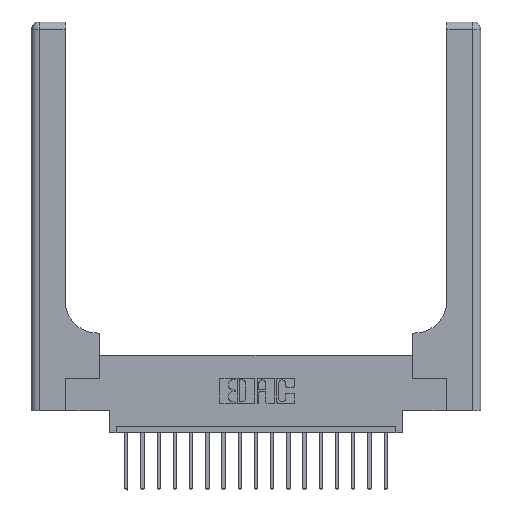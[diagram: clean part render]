
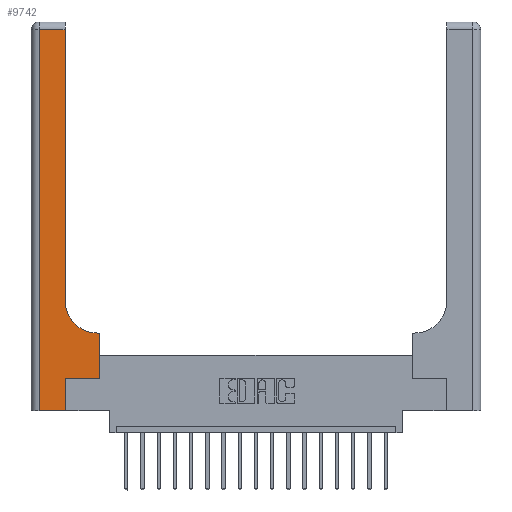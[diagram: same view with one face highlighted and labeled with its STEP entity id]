
A CAD part, top view. The second image highlights one B-rep face of the part: STEP entity #9742.
In plain terms, the highlighted planar face has unit normal (0, 0, 1).
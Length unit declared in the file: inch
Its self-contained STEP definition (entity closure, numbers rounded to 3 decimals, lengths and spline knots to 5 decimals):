
#14 = ORIENTED_EDGE ( 'NONE', *, *, #11265, .T. ) ;
#699 = DIRECTION ( 'NONE',  ( 0., 1., 0. ) ) ;
#896 = EDGE_LOOP ( 'NONE', ( #10444, #14141, #12593, #3415, #11266, #14292, #16196, #1144, #14 ) ) ;
#1080 = CARTESIAN_POINT ( 'NONE',  ( 0.265, 0.25, 0.37 ) ) ;
#1144 = ORIENTED_EDGE ( 'NONE', *, *, #6530, .T. ) ;
#1337 = VERTEX_POINT ( 'NONE', #7347 ) ;
#1409 = DIRECTION ( 'NONE',  ( 0., 1., 0. ) ) ;
#1794 = LINE ( 'NONE', #13833, #18723 ) ;
#1955 = CARTESIAN_POINT ( 'NONE',  ( 0.265, 0.25, 0.37 ) ) ;
#2036 = DIRECTION ( 'NONE',  ( -1., 0., 0. ) ) ;
#2071 = CARTESIAN_POINT ( 'NONE',  ( 0.26, 0.85, 0.37 ) ) ;
#2111 = LINE ( 'NONE', #3365, #17397 ) ;
#2700 = DIRECTION ( 'NONE',  ( 1., 0., 0. ) ) ;
#2970 = DIRECTION ( 'NONE',  ( 0., 1., 0. ) ) ;
#3365 = CARTESIAN_POINT ( 'NONE',  ( 0.528, 0.25, 0.37 ) ) ;
#3415 = ORIENTED_EDGE ( 'NONE', *, *, #11707, .T. ) ;
#3661 = LINE ( 'NONE', #10349, #5265 ) ;
#3766 = VECTOR ( 'NONE', #2700, 39.37008 ) ;
#4143 = EDGE_CURVE ( 'NONE', #1337, #18345, #2111, .T. ) ;
#4400 = CARTESIAN_POINT ( 'NONE',  ( 0.26, 2.94, 0.37 ) ) ;
#4460 = CIRCLE ( 'NONE', #9189, 0.25 ) ;
#4573 = LINE ( 'NONE', #12060, #5502 ) ;
#4612 = DIRECTION ( 'NONE',  ( 1., 0., 0. ) ) ;
#5010 = EDGE_CURVE ( 'NONE', #18431, #18228, #11331, .T. ) ;
#5265 = VECTOR ( 'NONE', #2970, 39.37008 ) ;
#5502 = VECTOR ( 'NONE', #13652, 39.37008 ) ;
#5650 = VERTEX_POINT ( 'NONE', #1080 ) ;
#5975 = EDGE_CURVE ( 'NONE', #5650, #1337, #9166, .T. ) ;
#6398 = CARTESIAN_POINT ( 'NONE',  ( 0.528, 0.6, 0.37 ) ) ;
#6530 = EDGE_CURVE ( 'NONE', #18345, #8696, #1794, .T. ) ;
#7207 = VERTEX_POINT ( 'NONE', #2071 ) ;
#7347 = CARTESIAN_POINT ( 'NONE',  ( 0.528, 0.25, 0.37 ) ) ;
#7786 = DIRECTION ( 'NONE',  ( -1., 0., 0. ) ) ;
#7935 = DIRECTION ( 'NONE',  ( 0., 0., -1. ) ) ;
#8696 = VERTEX_POINT ( 'NONE', #18028 ) ;
#8788 = EDGE_CURVE ( 'NONE', #7207, #14995, #3661, .T. ) ;
#9166 = LINE ( 'NONE', #1955, #10111 ) ;
#9174 = PLANE ( 'NONE',  #14900 ) ;
#9189 = AXIS2_PLACEMENT_3D ( 'NONE', #11883, #16386, #4612 ) ;
#9742 = ADVANCED_FACE ( 'NONE', ( #14523 ), #9174, .F. ) ;
#10111 = VECTOR ( 'NONE', #12582, 39.37008 ) ;
#10155 = CARTESIAN_POINT ( 'NONE',  ( 0.06, 2.94, 0.37 ) ) ;
#10349 = CARTESIAN_POINT ( 'NONE',  ( 0.26, 3., 0.37 ) ) ;
#10444 = ORIENTED_EDGE ( 'NONE', *, *, #8788, .T. ) ;
#10615 = VECTOR ( 'NONE', #13800, 39.37008 ) ;
#11148 = CARTESIAN_POINT ( 'NONE',  ( 0., 3., 0.37 ) ) ;
#11265 = EDGE_CURVE ( 'NONE', #8696, #7207, #4460, .T. ) ;
#11266 = ORIENTED_EDGE ( 'NONE', *, *, #18206, .T. ) ;
#11331 = LINE ( 'NONE', #12019, #10615 ) ;
#11529 = VERTEX_POINT ( 'NONE', #13926 ) ;
#11707 = EDGE_CURVE ( 'NONE', #18228, #11529, #14044, .T. ) ;
#11883 = CARTESIAN_POINT ( 'NONE',  ( 0.51, 0.85, 0.37 ) ) ;
#12019 = CARTESIAN_POINT ( 'NONE',  ( 0.06, 3., 0.37 ) ) ;
#12060 = CARTESIAN_POINT ( 'NONE',  ( 0., 2.94, 0.37 ) ) ;
#12582 = DIRECTION ( 'NONE',  ( 1., 0., 0. ) ) ;
#12593 = ORIENTED_EDGE ( 'NONE', *, *, #5010, .T. ) ;
#12853 = VECTOR ( 'NONE', #1409, 39.37008 ) ;
#13046 = CARTESIAN_POINT ( 'NONE',  ( 0., 0., 0.37 ) ) ;
#13652 = DIRECTION ( 'NONE',  ( -1., 0., 0. ) ) ;
#13800 = DIRECTION ( 'NONE',  ( 0., -1., 0. ) ) ;
#13833 = CARTESIAN_POINT ( 'NONE',  ( 0.26, 0.6, 0.37 ) ) ;
#13926 = CARTESIAN_POINT ( 'NONE',  ( 0.265, 0., 0.37 ) ) ;
#14044 = LINE ( 'NONE', #13046, #3766 ) ;
#14141 = ORIENTED_EDGE ( 'NONE', *, *, #14403, .T. ) ;
#14292 = ORIENTED_EDGE ( 'NONE', *, *, #5975, .T. ) ;
#14403 = EDGE_CURVE ( 'NONE', #14995, #18431, #4573, .T. ) ;
#14523 = FACE_OUTER_BOUND ( 'NONE', #896, .T. ) ;
#14701 = CARTESIAN_POINT ( 'NONE',  ( 0.265, 0., 0.37 ) ) ;
#14900 = AXIS2_PLACEMENT_3D ( 'NONE', #11148, #7935, #2036 ) ;
#14995 = VERTEX_POINT ( 'NONE', #4400 ) ;
#15112 = CARTESIAN_POINT ( 'NONE',  ( 0.06, 0., 0.37 ) ) ;
#15382 = LINE ( 'NONE', #14701, #12853 ) ;
#16196 = ORIENTED_EDGE ( 'NONE', *, *, #4143, .T. ) ;
#16386 = DIRECTION ( 'NONE',  ( 0., 0., -1. ) ) ;
#17397 = VECTOR ( 'NONE', #699, 39.37008 ) ;
#18028 = CARTESIAN_POINT ( 'NONE',  ( 0.51, 0.6, 0.37 ) ) ;
#18206 = EDGE_CURVE ( 'NONE', #11529, #5650, #15382, .T. ) ;
#18228 = VERTEX_POINT ( 'NONE', #15112 ) ;
#18345 = VERTEX_POINT ( 'NONE', #6398 ) ;
#18431 = VERTEX_POINT ( 'NONE', #10155 ) ;
#18723 = VECTOR ( 'NONE', #7786, 39.37008 ) ;
